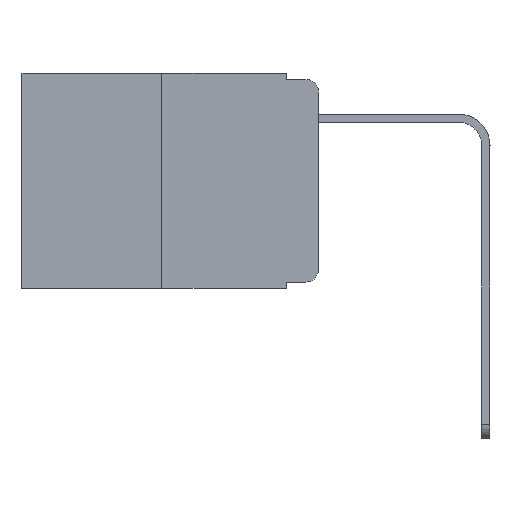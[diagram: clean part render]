
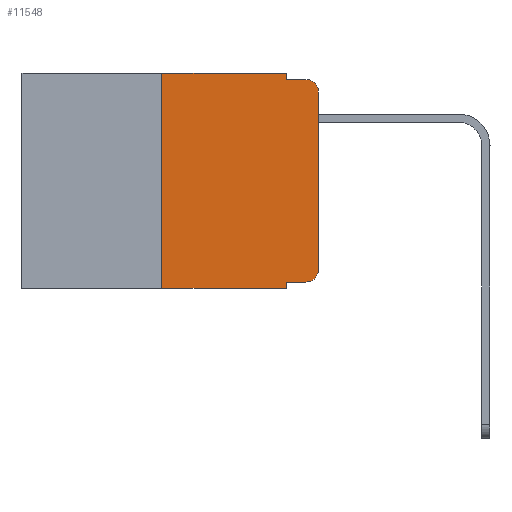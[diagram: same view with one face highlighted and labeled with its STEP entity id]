
A CAD part, left-side view. The second image highlights one B-rep face of the part: STEP entity #11548.
In plain terms, the highlighted planar face has unit normal (-1, 0, 0).
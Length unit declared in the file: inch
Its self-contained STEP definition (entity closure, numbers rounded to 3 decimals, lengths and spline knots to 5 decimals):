
#35 = EDGE_LOOP ( 'NONE', ( #654, #19384, #5482, #4723, #18400, #17149, #16314, #8562, #8119, #1424 ) ) ;
#173 = CARTESIAN_POINT ( 'NONE',  ( 0., 0.051, -0.333 ) ) ;
#192 = EDGE_CURVE ( 'NONE', #13181, #16199, #15481, .T. ) ;
#411 = DIRECTION ( 'NONE',  ( 0., 0., -1. ) ) ;
#493 = CARTESIAN_POINT ( 'NONE',  ( 0., 0.051, 0. ) ) ;
#654 = ORIENTED_EDGE ( 'NONE', *, *, #19632, .T. ) ;
#1162 = VECTOR ( 'NONE', #2896, 39.37008 ) ;
#1176 = CARTESIAN_POINT ( 'NONE',  ( 0., 0.25, 0. ) ) ;
#1186 = CARTESIAN_POINT ( 'NONE',  ( 0., 0.051, -0.343 ) ) ;
#1424 = ORIENTED_EDGE ( 'NONE', *, *, #9486, .T. ) ;
#1593 = CARTESIAN_POINT ( 'NONE',  ( 0., 0.051, 0. ) ) ;
#1992 = EDGE_CURVE ( 'NONE', #16199, #16263, #11008, .T. ) ;
#2447 = AXIS2_PLACEMENT_3D ( 'NONE', #15266, #17006, #8647 ) ;
#2750 = VERTEX_POINT ( 'NONE', #13225 ) ;
#2896 = DIRECTION ( 'NONE',  ( 0., -1., 0. ) ) ;
#2988 = EDGE_CURVE ( 'NONE', #13181, #13922, #5027, .T. ) ;
#3383 = CARTESIAN_POINT ( 'NONE',  ( 0., 0., 0. ) ) ;
#3439 = VERTEX_POINT ( 'NONE', #7989 ) ;
#4070 = LINE ( 'NONE', #1593, #12823 ) ;
#4223 = CARTESIAN_POINT ( 'NONE',  ( 0., 0.02, -0.313 ) ) ;
#4560 = DIRECTION ( 'NONE',  ( -1., 0., 0. ) ) ;
#4723 = ORIENTED_EDGE ( 'NONE', *, *, #12602, .F. ) ;
#5027 = LINE ( 'NONE', #12567, #17704 ) ;
#5074 = EDGE_CURVE ( 'NONE', #3439, #13558, #18354, .T. ) ;
#5355 = EDGE_CURVE ( 'NONE', #19735, #20954, #13915, .T. ) ;
#5482 = ORIENTED_EDGE ( 'NONE', *, *, #11446, .F. ) ;
#5655 = VECTOR ( 'NONE', #6487, 39.37008 ) ;
#6207 = VECTOR ( 'NONE', #411, 39.37008 ) ;
#6487 = DIRECTION ( 'NONE',  ( 0., 0., 1. ) ) ;
#6585 = DIRECTION ( 'NONE',  ( 0., 0., 1. ) ) ;
#6587 = DIRECTION ( 'NONE',  ( 0., -1., 0. ) ) ;
#6768 = VECTOR ( 'NONE', #17543, 39.37008 ) ;
#6975 = CARTESIAN_POINT ( 'NONE',  ( 0., 0.051, 0. ) ) ;
#7257 = LINE ( 'NONE', #493, #6207 ) ;
#7465 = CARTESIAN_POINT ( 'NONE',  ( 0., 0.25, -0.343 ) ) ;
#7652 = CARTESIAN_POINT ( 'NONE',  ( 0., 0.051, -0.333 ) ) ;
#7989 = CARTESIAN_POINT ( 'NONE',  ( 0., 0., -0.03 ) ) ;
#8119 = ORIENTED_EDGE ( 'NONE', *, *, #5355, .T. ) ;
#8562 = ORIENTED_EDGE ( 'NONE', *, *, #10486, .F. ) ;
#8647 = DIRECTION ( 'NONE',  ( 0., 0., -1. ) ) ;
#9195 = DIRECTION ( 'NONE',  ( 0., 0., -1. ) ) ;
#9486 = EDGE_CURVE ( 'NONE', #20954, #2750, #12165, .T. ) ;
#10486 = EDGE_CURVE ( 'NONE', #19735, #13922, #4070, .T. ) ;
#10787 = DIRECTION ( 'NONE',  ( -1., 0., 0. ) ) ;
#11008 = LINE ( 'NONE', #12943, #1162 ) ;
#11290 = AXIS2_PLACEMENT_3D ( 'NONE', #4223, #10787, #9195 ) ;
#11446 = EDGE_CURVE ( 'NONE', #20471, #13558, #12707, .T. ) ;
#11548 = ADVANCED_FACE ( 'NONE', ( #20488 ), #15402, .F. ) ;
#12165 = CIRCLE ( 'NONE', #11290, 0.02 ) ;
#12548 = CARTESIAN_POINT ( 'NONE',  ( 0., 0.051, -0.01 ) ) ;
#12567 = CARTESIAN_POINT ( 'NONE',  ( 0., 0.473, -0.343 ) ) ;
#12602 = EDGE_CURVE ( 'NONE', #16263, #20471, #7257, .T. ) ;
#12707 = LINE ( 'NONE', #12548, #6768 ) ;
#12823 = VECTOR ( 'NONE', #14958, 39.37008 ) ;
#12909 = AXIS2_PLACEMENT_3D ( 'NONE', #19301, #4560, #20964 ) ;
#12943 = CARTESIAN_POINT ( 'NONE',  ( 0., 0.473, 0. ) ) ;
#13181 = VERTEX_POINT ( 'NONE', #7465 ) ;
#13225 = CARTESIAN_POINT ( 'NONE',  ( 0., 0., -0.313 ) ) ;
#13558 = VERTEX_POINT ( 'NONE', #18221 ) ;
#13915 = LINE ( 'NONE', #7652, #20411 ) ;
#13922 = VERTEX_POINT ( 'NONE', #1186 ) ;
#14920 = CARTESIAN_POINT ( 'NONE',  ( 0., 0.25, 0. ) ) ;
#14958 = DIRECTION ( 'NONE',  ( 0., 0., -1. ) ) ;
#15266 = CARTESIAN_POINT ( 'NONE',  ( 0., 0.473, 0. ) ) ;
#15402 = PLANE ( 'NONE',  #2447 ) ;
#15481 = LINE ( 'NONE', #1176, #5655 ) ;
#16199 = VERTEX_POINT ( 'NONE', #14920 ) ;
#16263 = VERTEX_POINT ( 'NONE', #6975 ) ;
#16314 = ORIENTED_EDGE ( 'NONE', *, *, #2988, .T. ) ;
#17006 = DIRECTION ( 'NONE',  ( 1., 0., 0. ) ) ;
#17149 = ORIENTED_EDGE ( 'NONE', *, *, #192, .F. ) ;
#17165 = CARTESIAN_POINT ( 'NONE',  ( 0., 0.051, -0.01 ) ) ;
#17543 = DIRECTION ( 'NONE',  ( 0., -1., 0. ) ) ;
#17704 = VECTOR ( 'NONE', #6587, 39.37008 ) ;
#18221 = CARTESIAN_POINT ( 'NONE',  ( 0., 0.02, -0.01 ) ) ;
#18354 = CIRCLE ( 'NONE', #12909, 0.02 ) ;
#18400 = ORIENTED_EDGE ( 'NONE', *, *, #1992, .F. ) ;
#19195 = DIRECTION ( 'NONE',  ( 0., -1., 0. ) ) ;
#19301 = CARTESIAN_POINT ( 'NONE',  ( 0., 0.02, -0.03 ) ) ;
#19384 = ORIENTED_EDGE ( 'NONE', *, *, #5074, .T. ) ;
#19632 = EDGE_CURVE ( 'NONE', #2750, #3439, #20305, .T. ) ;
#19735 = VERTEX_POINT ( 'NONE', #173 ) ;
#20305 = LINE ( 'NONE', #3383, #21315 ) ;
#20401 = CARTESIAN_POINT ( 'NONE',  ( 0., 0.02, -0.333 ) ) ;
#20411 = VECTOR ( 'NONE', #19195, 39.37008 ) ;
#20471 = VERTEX_POINT ( 'NONE', #17165 ) ;
#20488 = FACE_OUTER_BOUND ( 'NONE', #35, .T. ) ;
#20954 = VERTEX_POINT ( 'NONE', #20401 ) ;
#20964 = DIRECTION ( 'NONE',  ( 0., 0., -1. ) ) ;
#21315 = VECTOR ( 'NONE', #6585, 39.37008 ) ;
